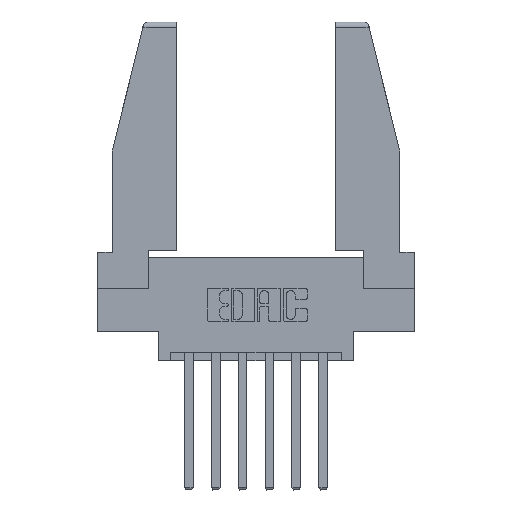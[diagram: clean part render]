
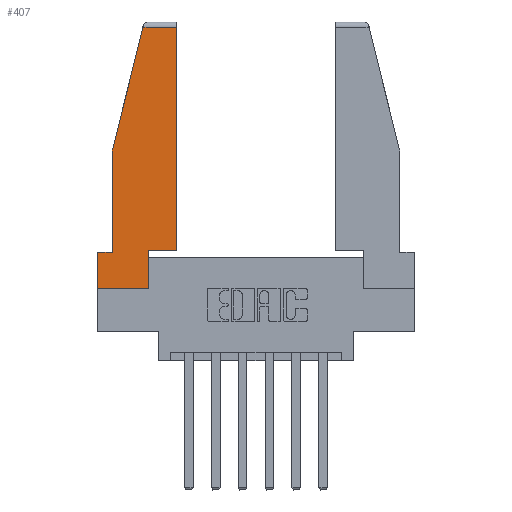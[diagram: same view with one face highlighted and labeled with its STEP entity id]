
A CAD part, top view. The second image highlights one B-rep face of the part: STEP entity #407.
In plain terms, the highlighted planar face has unit normal (0, 0, 1).
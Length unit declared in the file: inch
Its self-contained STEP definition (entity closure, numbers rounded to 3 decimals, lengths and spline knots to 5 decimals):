
#21 = VERTEX_POINT ( 'NONE', #10375 ) ;
#51 = ORIENTED_EDGE ( 'NONE', *, *, #10292, .T. ) ;
#336 = VECTOR ( 'NONE', #5149, 39.37008 ) ;
#407 = ADVANCED_FACE ( 'NONE', ( #10927 ), #1274, .T. ) ;
#412 = CARTESIAN_POINT ( 'NONE',  ( 0., 0.21, 0. ) ) ;
#451 = VERTEX_POINT ( 'NONE', #3744 ) ;
#511 = EDGE_LOOP ( 'NONE', ( #985, #7271, #3015, #10840, #4415, #1946, #51, #11483, #6074 ) ) ;
#737 = CARTESIAN_POINT ( 'NONE',  ( 0., 1.52, 0. ) ) ;
#985 = ORIENTED_EDGE ( 'NONE', *, *, #7301, .T. ) ;
#1171 = LINE ( 'NONE', #8178, #4024 ) ;
#1274 = PLANE ( 'NONE',  #8801 ) ;
#1292 = CARTESIAN_POINT ( 'NONE',  ( 0.297, 0., 0. ) ) ;
#1407 = VECTOR ( 'NONE', #7739, 39.37008 ) ;
#1816 = EDGE_CURVE ( 'NONE', #5697, #451, #8957, .T. ) ;
#1946 = ORIENTED_EDGE ( 'NONE', *, *, #7940, .T. ) ;
#1947 = EDGE_CURVE ( 'NONE', #9108, #7167, #6590, .T. ) ;
#2097 = DIRECTION ( 'NONE',  ( 1., 0., 0. ) ) ;
#2612 = EDGE_CURVE ( 'NONE', #21, #2873, #9761, .T. ) ;
#2675 = DIRECTION ( 'NONE',  ( 0., 1., 0. ) ) ;
#2702 = CARTESIAN_POINT ( 'NONE',  ( 0.086, 0.8, 0. ) ) ;
#2721 = DIRECTION ( 'NONE',  ( -0.239, -0.971, 0. ) ) ;
#2873 = VERTEX_POINT ( 'NONE', #4630 ) ;
#2984 = DIRECTION ( 'NONE',  ( 0., -1., 0. ) ) ;
#3015 = ORIENTED_EDGE ( 'NONE', *, *, #7236, .T. ) ;
#3278 = VERTEX_POINT ( 'NONE', #9311 ) ;
#3744 = CARTESIAN_POINT ( 'NONE',  ( 0.2636, 1.52, 0. ) ) ;
#3794 = DIRECTION ( 'NONE',  ( 0., -1., 0. ) ) ;
#4024 = VECTOR ( 'NONE', #2675, 39.37008 ) ;
#4156 = VECTOR ( 'NONE', #2097, 39.37008 ) ;
#4325 = LINE ( 'NONE', #9256, #8628 ) ;
#4368 = CARTESIAN_POINT ( 'NONE',  ( 0.461, 0.223, 0. ) ) ;
#4411 = CARTESIAN_POINT ( 'NONE',  ( 0., 0., 0. ) ) ;
#4415 = ORIENTED_EDGE ( 'NONE', *, *, #6484, .T. ) ;
#4499 = VECTOR ( 'NONE', #9017, 39.37008 ) ;
#4630 = CARTESIAN_POINT ( 'NONE',  ( 0.086, 0.21, 0. ) ) ;
#4887 = VECTOR ( 'NONE', #3794, 39.37008 ) ;
#5149 = DIRECTION ( 'NONE',  ( 1., 0., 0. ) ) ;
#5262 = LINE ( 'NONE', #1292, #1407 ) ;
#5589 = CARTESIAN_POINT ( 'NONE',  ( 0.297, 0.223, 0. ) ) ;
#5604 = VECTOR ( 'NONE', #2721, 39.37008 ) ;
#5697 = VERTEX_POINT ( 'NONE', #8952 ) ;
#6074 = ORIENTED_EDGE ( 'NONE', *, *, #1947, .T. ) ;
#6092 = DIRECTION ( 'NONE',  ( 1., 0., 0. ) ) ;
#6301 = LINE ( 'NONE', #7292, #5604 ) ;
#6484 = EDGE_CURVE ( 'NONE', #2873, #6650, #4325, .T. ) ;
#6590 = LINE ( 'NONE', #5589, #4156 ) ;
#6650 = VERTEX_POINT ( 'NONE', #10322 ) ;
#7167 = VERTEX_POINT ( 'NONE', #4368 ) ;
#7185 = VERTEX_POINT ( 'NONE', #4411 ) ;
#7236 = EDGE_CURVE ( 'NONE', #451, #21, #6301, .T. ) ;
#7271 = ORIENTED_EDGE ( 'NONE', *, *, #1816, .T. ) ;
#7292 = CARTESIAN_POINT ( 'NONE',  ( 0.271, 1.55, 0. ) ) ;
#7301 = EDGE_CURVE ( 'NONE', #7167, #5697, #1171, .T. ) ;
#7681 = DIRECTION ( 'NONE',  ( 0., 0., 1. ) ) ;
#7739 = DIRECTION ( 'NONE',  ( 0., 1., 0. ) ) ;
#7865 = LINE ( 'NONE', #9805, #336 ) ;
#7940 = EDGE_CURVE ( 'NONE', #6650, #7185, #8305, .T. ) ;
#8158 = VECTOR ( 'NONE', #2984, 39.37008 ) ;
#8178 = CARTESIAN_POINT ( 'NONE',  ( 0.461, 0.223, 0. ) ) ;
#8305 = LINE ( 'NONE', #412, #8158 ) ;
#8628 = VECTOR ( 'NONE', #10056, 39.37008 ) ;
#8801 = AXIS2_PLACEMENT_3D ( 'NONE', #9489, #7681, #6092 ) ;
#8952 = CARTESIAN_POINT ( 'NONE',  ( 0.461, 1.52, 0. ) ) ;
#8957 = LINE ( 'NONE', #737, #4499 ) ;
#9017 = DIRECTION ( 'NONE',  ( -1., 0., 0. ) ) ;
#9108 = VERTEX_POINT ( 'NONE', #9563 ) ;
#9256 = CARTESIAN_POINT ( 'NONE',  ( 0., 0.21, 0. ) ) ;
#9311 = CARTESIAN_POINT ( 'NONE',  ( 0.297, 0., 0. ) ) ;
#9489 = CARTESIAN_POINT ( 'NONE',  ( 0., 0., 0. ) ) ;
#9563 = CARTESIAN_POINT ( 'NONE',  ( 0.297, 0.223, 0. ) ) ;
#9761 = LINE ( 'NONE', #2702, #4887 ) ;
#9805 = CARTESIAN_POINT ( 'NONE',  ( 0., 0., 0. ) ) ;
#10056 = DIRECTION ( 'NONE',  ( -1., 0., 0. ) ) ;
#10292 = EDGE_CURVE ( 'NONE', #7185, #3278, #7865, .T. ) ;
#10322 = CARTESIAN_POINT ( 'NONE',  ( 0., 0.21, 0. ) ) ;
#10375 = CARTESIAN_POINT ( 'NONE',  ( 0.086, 0.8, 0. ) ) ;
#10840 = ORIENTED_EDGE ( 'NONE', *, *, #2612, .T. ) ;
#10862 = EDGE_CURVE ( 'NONE', #3278, #9108, #5262, .T. ) ;
#10927 = FACE_OUTER_BOUND ( 'NONE', #511, .T. ) ;
#11483 = ORIENTED_EDGE ( 'NONE', *, *, #10862, .T. ) ;
